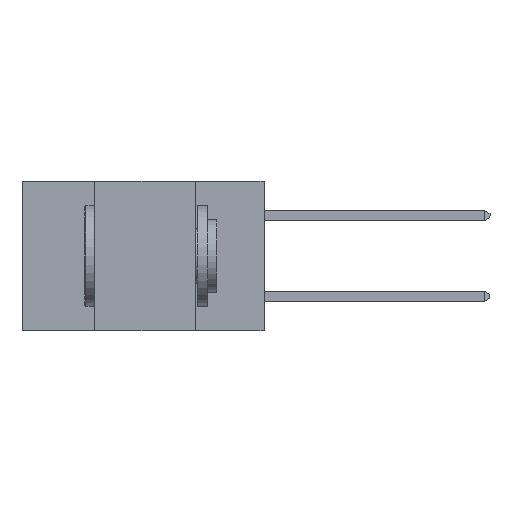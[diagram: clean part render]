
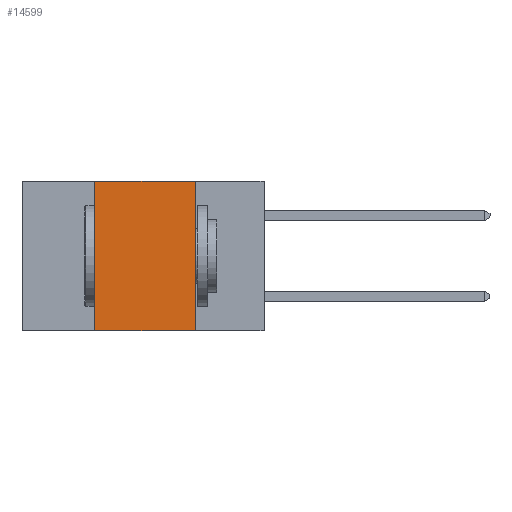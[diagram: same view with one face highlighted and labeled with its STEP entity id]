
A CAD part, left-side view. The second image highlights one B-rep face of the part: STEP entity #14599.
In plain terms, the highlighted planar face has unit normal (-1, 0, 0).
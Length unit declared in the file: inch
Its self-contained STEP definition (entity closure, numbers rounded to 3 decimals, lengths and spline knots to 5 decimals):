
#774 = CARTESIAN_POINT ( 'NONE',  ( 0., 0.42, 0. ) ) ;
#1007 = CARTESIAN_POINT ( 'NONE',  ( 0., 0.6, 0. ) ) ;
#1073 = VERTEX_POINT ( 'NONE', #13893 ) ;
#1074 = DIRECTION ( 'NONE',  ( 0., -1., 0. ) ) ;
#1252 = LINE ( 'NONE', #3590, #10051 ) ;
#2302 = ORIENTED_EDGE ( 'NONE', *, *, #13604, .T. ) ;
#2600 = VECTOR ( 'NONE', #14762, 39.37008 ) ;
#3132 = VERTEX_POINT ( 'NONE', #6867 ) ;
#3267 = DIRECTION ( 'NONE',  ( 0., -1., 0. ) ) ;
#3590 = CARTESIAN_POINT ( 'NONE',  ( 0., 0.42, 0. ) ) ;
#4460 = VECTOR ( 'NONE', #3267, 39.37008 ) ;
#4865 = LINE ( 'NONE', #15151, #13781 ) ;
#5387 = ORIENTED_EDGE ( 'NONE', *, *, #10671, .F. ) ;
#5895 = DIRECTION ( 'NONE',  ( 0., 0., -1. ) ) ;
#6867 = CARTESIAN_POINT ( 'NONE',  ( 0., 0.17, -0.37 ) ) ;
#7066 = VERTEX_POINT ( 'NONE', #12136 ) ;
#7507 = EDGE_LOOP ( 'NONE', ( #9488, #5387, #10719, #2302 ) ) ;
#7646 = VERTEX_POINT ( 'NONE', #774 ) ;
#7861 = CARTESIAN_POINT ( 'NONE',  ( 0., 0.17, 0. ) ) ;
#8216 = PLANE ( 'NONE',  #8685 ) ;
#8685 = AXIS2_PLACEMENT_3D ( 'NONE', #1007, #12835, #5895 ) ;
#9488 = ORIENTED_EDGE ( 'NONE', *, *, #9972, .F. ) ;
#9972 = EDGE_CURVE ( 'NONE', #1073, #3132, #12018, .T. ) ;
#10051 = VECTOR ( 'NONE', #12940, 39.37008 ) ;
#10671 = EDGE_CURVE ( 'NONE', #7646, #1073, #4865, .T. ) ;
#10719 = ORIENTED_EDGE ( 'NONE', *, *, #10730, .F. ) ;
#10730 = EDGE_CURVE ( 'NONE', #7066, #7646, #1252, .T. ) ;
#11078 = LINE ( 'NONE', #14903, #4460 ) ;
#11582 = FACE_OUTER_BOUND ( 'NONE', #7507, .T. ) ;
#12018 = LINE ( 'NONE', #7861, #2600 ) ;
#12136 = CARTESIAN_POINT ( 'NONE',  ( 0., 0.42, -0.37 ) ) ;
#12835 = DIRECTION ( 'NONE',  ( 1., 0., 0. ) ) ;
#12940 = DIRECTION ( 'NONE',  ( 0., 0., 1. ) ) ;
#13604 = EDGE_CURVE ( 'NONE', #7066, #3132, #11078, .T. ) ;
#13781 = VECTOR ( 'NONE', #1074, 39.37008 ) ;
#13893 = CARTESIAN_POINT ( 'NONE',  ( 0., 0.17, 0. ) ) ;
#14599 = ADVANCED_FACE ( 'NONE', ( #11582 ), #8216, .F. ) ;
#14762 = DIRECTION ( 'NONE',  ( 0., 0., -1. ) ) ;
#14903 = CARTESIAN_POINT ( 'NONE',  ( 0., 0.6, -0.37 ) ) ;
#15151 = CARTESIAN_POINT ( 'NONE',  ( 0., 0.6, 0. ) ) ;
